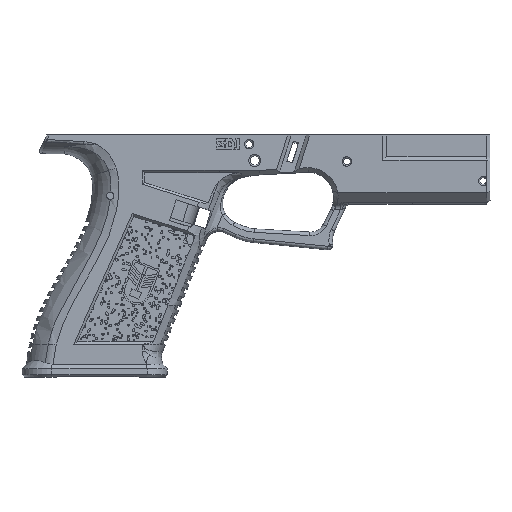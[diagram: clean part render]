
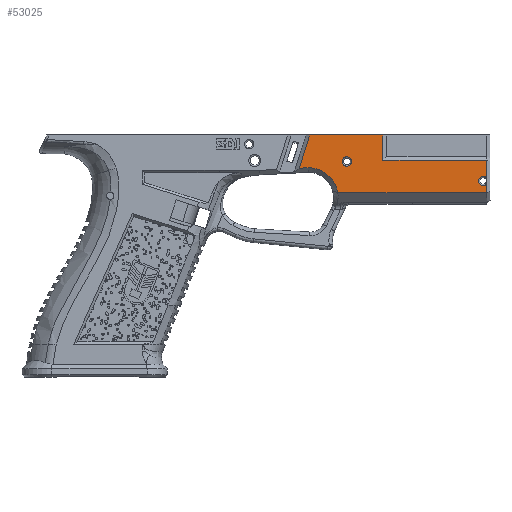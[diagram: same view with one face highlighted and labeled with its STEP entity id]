
A CAD part, front view. The second image highlights one B-rep face of the part: STEP entity #53025.
In plain terms, the highlighted planar face has unit normal (0, -1, 0).
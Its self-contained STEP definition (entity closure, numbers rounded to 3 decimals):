
#5873=FACE_BOUND('',#9894,.T.);
#6296=CIRCLE('',#56293,13.);
#6297=CIRCLE('',#56294,2.);
#6298=CIRCLE('',#56295,2.);
#6650=FACE_OUTER_BOUND('',#9893,.T.);
#9893=EDGE_LOOP('',(#35600,#35601,#35602,#35603,#35604,#35605,#35606,#35607,
#35608,#35609,#35610,#35611));
#9894=EDGE_LOOP('',(#35612));
#13588=LINE('',#66877,#16887);
#13610=LINE('',#69026,#16909);
#13611=LINE('',#69028,#16910);
#13612=LINE('',#69032,#16911);
#13613=LINE('',#69034,#16912);
#13614=LINE('',#69036,#16913);
#13615=LINE('',#69040,#16914);
#13616=LINE('',#69042,#16915);
#13617=LINE('',#69044,#16916);
#13618=LINE('',#69045,#16917);
#16887=VECTOR('',#57605,10.);
#16909=VECTOR('',#57639,10.);
#16910=VECTOR('',#57640,10.);
#16911=VECTOR('',#57643,10.);
#16912=VECTOR('',#57644,10.);
#16913=VECTOR('',#57645,10.);
#16914=VECTOR('',#57648,10.);
#16915=VECTOR('',#57649,10.);
#16916=VECTOR('',#57650,10.);
#16917=VECTOR('',#57651,10.);
#21476=VERTEX_POINT('',#66874);
#21477=VERTEX_POINT('',#66876);
#21572=VERTEX_POINT('',#69025);
#21573=VERTEX_POINT('',#69027);
#21574=VERTEX_POINT('',#69029);
#21575=VERTEX_POINT('',#69031);
#21576=VERTEX_POINT('',#69033);
#21577=VERTEX_POINT('',#69035);
#21578=VERTEX_POINT('',#69037);
#21579=VERTEX_POINT('',#69039);
#21580=VERTEX_POINT('',#69041);
#21581=VERTEX_POINT('',#69043);
#21582=VERTEX_POINT('',#69046);
#27041=EDGE_CURVE('',#21477,#21476,#13588,.T.);
#27141=EDGE_CURVE('',#21572,#21476,#13610,.T.);
#27142=EDGE_CURVE('',#21573,#21572,#13611,.T.);
#27143=EDGE_CURVE('',#21574,#21573,#6296,.T.);
#27144=EDGE_CURVE('',#21575,#21574,#13612,.T.);
#27145=EDGE_CURVE('',#21576,#21575,#13613,.T.);
#27146=EDGE_CURVE('',#21577,#21576,#13614,.T.);
#27147=EDGE_CURVE('',#21578,#21577,#6297,.T.);
#27148=EDGE_CURVE('',#21579,#21578,#13615,.T.);
#27149=EDGE_CURVE('',#21579,#21580,#13616,.T.);
#27150=EDGE_CURVE('',#21580,#21581,#13617,.T.);
#27151=EDGE_CURVE('',#21477,#21581,#13618,.T.);
#27152=EDGE_CURVE('',#21582,#21582,#6298,.T.);
#35600=ORIENTED_EDGE('',*,*,#27041,.T.);
#35601=ORIENTED_EDGE('',*,*,#27141,.F.);
#35602=ORIENTED_EDGE('',*,*,#27142,.F.);
#35603=ORIENTED_EDGE('',*,*,#27143,.F.);
#35604=ORIENTED_EDGE('',*,*,#27144,.F.);
#35605=ORIENTED_EDGE('',*,*,#27145,.F.);
#35606=ORIENTED_EDGE('',*,*,#27146,.F.);
#35607=ORIENTED_EDGE('',*,*,#27147,.F.);
#35608=ORIENTED_EDGE('',*,*,#27148,.F.);
#35609=ORIENTED_EDGE('',*,*,#27149,.T.);
#35610=ORIENTED_EDGE('',*,*,#27150,.T.);
#35611=ORIENTED_EDGE('',*,*,#27151,.F.);
#35612=ORIENTED_EDGE('',*,*,#27152,.F.);
#52087=PLANE('',#56292);
#53025=ADVANCED_FACE('',(#6650,#5873),#52087,.F.);
#56292=AXIS2_PLACEMENT_3D('',#69024,#57637,#57638);
#56293=AXIS2_PLACEMENT_3D('',#69030,#57641,#57642);
#56294=AXIS2_PLACEMENT_3D('',#69038,#57646,#57647);
#56295=AXIS2_PLACEMENT_3D('',#69047,#57652,#57653);
#57605=DIRECTION('',(-1.,0.,0.));
#57637=DIRECTION('center_axis',(0.,1.,0.));
#57638=DIRECTION('ref_axis',(0.,0.,
1.));
#57639=DIRECTION('',(0.301,0.,0.954));
#57640=DIRECTION('',(-0.999,0.,-0.055));
#57641=DIRECTION('center_axis',(0.,-1.,0.));
#57642=DIRECTION('ref_axis',(0.892,0.,-0.452));
#57643=DIRECTION('',(-1.,0.,0.));
#57644=DIRECTION('',(-1.,0.,0.));
#57645=DIRECTION('',(0.,0.,-1.));
#57646=DIRECTION('center_axis',(0.,-1.,0.));
#57647=DIRECTION('ref_axis',(-1.,0.,0.));
#57648=DIRECTION('',(0.,0.,-1.));
#57649=DIRECTION('',(-1.,0.,0.));
#57650=DIRECTION('',(-1.,0.,0.));
#57651=DIRECTION('',(0.,0.,-1.));
#57652=DIRECTION('center_axis',(0.,-1.,0.));
#57653=DIRECTION('ref_axis',(1.,0.,0.));
#66874=CARTESIAN_POINT('',(80.915,-135.077,16.843));
#66876=CARTESIAN_POINT('',(112.635,-135.077,16.843));
#66877=CARTESIAN_POINT('',(27.342,-135.077,16.843));
#69024=CARTESIAN_POINT('Origin',(82.31,-135.077,16.95));
#69025=CARTESIAN_POINT('',(76.374,-135.077,2.443));
#69026=CARTESIAN_POINT('',(80.837,-135.077,16.595));
#69027=CARTESIAN_POINT('',(80.217,-135.077,2.654));
#69028=CARTESIAN_POINT('',(81.633,-135.077,2.731));
#69029=CARTESIAN_POINT('',(93.078,-135.077,-8.096));
#69030=CARTESIAN_POINT('Origin',(80.274,-135.077,-10.346));
#69031=CARTESIAN_POINT('',(125.385,-135.077,-8.097));
#69032=CARTESIAN_POINT('',(89.618,-135.077,-8.096));
#69033=CARTESIAN_POINT('',(157.635,-135.077,-8.097));
#69034=CARTESIAN_POINT('',(68.618,-135.077,-8.097));
#69035=CARTESIAN_POINT('',(157.635,-135.077,-4.419));
#69036=CARTESIAN_POINT('',(157.635,-135.077,-9.397));
#69037=CARTESIAN_POINT('',(157.635,-135.077,-1.774));
#69038=CARTESIAN_POINT('Origin',(156.135,-135.077,-3.096));
#69039=CARTESIAN_POINT('',(157.635,-135.077,5.957));
#69040=CARTESIAN_POINT('',(157.635,-135.077,-9.397));
#69041=CARTESIAN_POINT('',(125.385,-135.077,5.957));
#69042=CARTESIAN_POINT('',(84.549,-135.077,5.957));
#69043=CARTESIAN_POINT('',(112.635,-135.077,5.957));
#69044=CARTESIAN_POINT('',(105.549,-135.077,5.957));
#69045=CARTESIAN_POINT('',(112.635,-135.077,17.203));
#69046=CARTESIAN_POINT('',(97.018,-135.077,3.35));
#69047=CARTESIAN_POINT('Origin',(97.018,-135.077,5.35));
